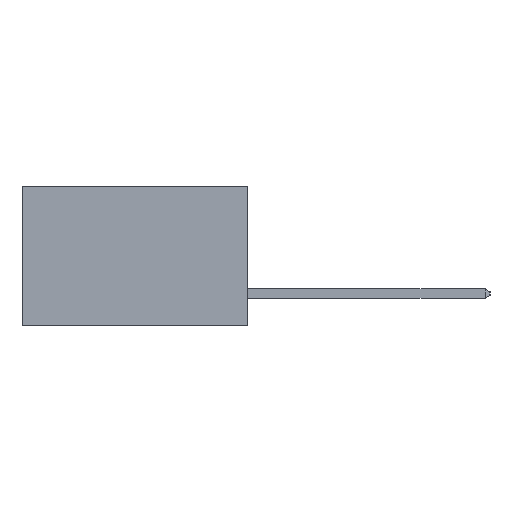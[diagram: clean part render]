
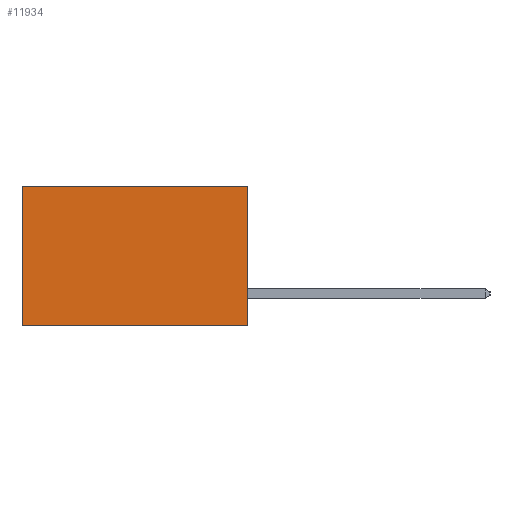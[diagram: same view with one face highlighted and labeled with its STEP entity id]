
A CAD part, left-side view. The second image highlights one B-rep face of the part: STEP entity #11934.
In plain terms, the highlighted planar face has unit normal (-1, 0, 0).
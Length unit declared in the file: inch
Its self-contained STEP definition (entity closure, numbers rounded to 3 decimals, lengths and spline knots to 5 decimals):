
#206 = AXIS2_PLACEMENT_3D ( 'NONE', #8187, #1195, #9389 ) ;
#240 = CARTESIAN_POINT ( 'NONE',  ( 0.2615, 0.6, 0. ) ) ;
#1131 = DIRECTION ( 'NONE',  ( 0., 0., -1. ) ) ;
#1195 = DIRECTION ( 'NONE',  ( 1., 0., 0. ) ) ;
#1344 = CARTESIAN_POINT ( 'NONE',  ( 0.2615, 0.6, -0.37 ) ) ;
#2434 = ORIENTED_EDGE ( 'NONE', *, *, #7794, .T. ) ;
#2770 = VECTOR ( 'NONE', #9215, 39.37008 ) ;
#2819 = CARTESIAN_POINT ( 'NONE',  ( 0.2615, 0., -0.37 ) ) ;
#3728 = LINE ( 'NONE', #13415, #6500 ) ;
#4478 = EDGE_CURVE ( 'NONE', #8205, #11568, #8662, .T. ) ;
#5042 = VECTOR ( 'NONE', #6449, 39.37008 ) ;
#5547 = CARTESIAN_POINT ( 'NONE',  ( 0.2615, 0., -0.37 ) ) ;
#5779 = LINE ( 'NONE', #6387, #5042 ) ;
#5843 = PLANE ( 'NONE',  #206 ) ;
#6387 = CARTESIAN_POINT ( 'NONE',  ( 0.2615, 0., -0.37 ) ) ;
#6449 = DIRECTION ( 'NONE',  ( 0., 1., 0. ) ) ;
#6500 = VECTOR ( 'NONE', #13502, 39.37008 ) ;
#6850 = CARTESIAN_POINT ( 'NONE',  ( 0.2615, 0., 0. ) ) ;
#7794 = EDGE_CURVE ( 'NONE', #13620, #14201, #3728, .T. ) ;
#8187 = CARTESIAN_POINT ( 'NONE',  ( 0.2615, 0., -0.37 ) ) ;
#8205 = VERTEX_POINT ( 'NONE', #8490 ) ;
#8322 = ORIENTED_EDGE ( 'NONE', *, *, #4478, .F. ) ;
#8473 = ORIENTED_EDGE ( 'NONE', *, *, #14666, .T. ) ;
#8490 = CARTESIAN_POINT ( 'NONE',  ( 0.2615, 0., 0. ) ) ;
#8662 = LINE ( 'NONE', #5547, #14268 ) ;
#9190 = ORIENTED_EDGE ( 'NONE', *, *, #13140, .F. ) ;
#9215 = DIRECTION ( 'NONE',  ( 0., 1., 0. ) ) ;
#9389 = DIRECTION ( 'NONE',  ( 0., 0., -1. ) ) ;
#10342 = EDGE_LOOP ( 'NONE', ( #2434, #9190, #8322, #8473 ) ) ;
#10374 = FACE_OUTER_BOUND ( 'NONE', #10342, .T. ) ;
#11568 = VERTEX_POINT ( 'NONE', #2819 ) ;
#11934 = ADVANCED_FACE ( 'NONE', ( #10374 ), #5843, .F. ) ;
#12069 = LINE ( 'NONE', #6850, #2770 ) ;
#13140 = EDGE_CURVE ( 'NONE', #11568, #14201, #5779, .T. ) ;
#13415 = CARTESIAN_POINT ( 'NONE',  ( 0.2615, 0.6, -0.37 ) ) ;
#13502 = DIRECTION ( 'NONE',  ( 0., 0., -1. ) ) ;
#13620 = VERTEX_POINT ( 'NONE', #240 ) ;
#14201 = VERTEX_POINT ( 'NONE', #1344 ) ;
#14268 = VECTOR ( 'NONE', #1131, 39.37008 ) ;
#14666 = EDGE_CURVE ( 'NONE', #8205, #13620, #12069, .T. ) ;
